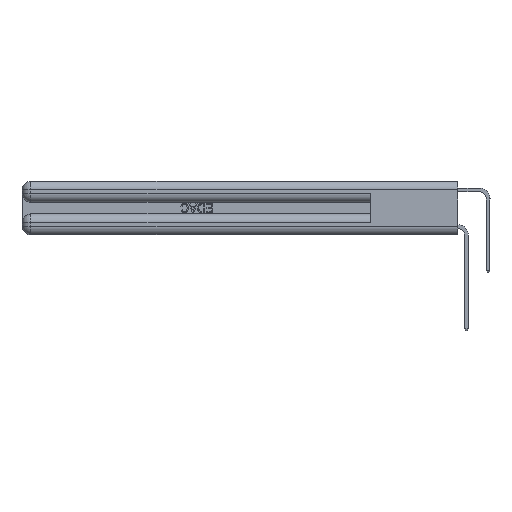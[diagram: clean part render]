
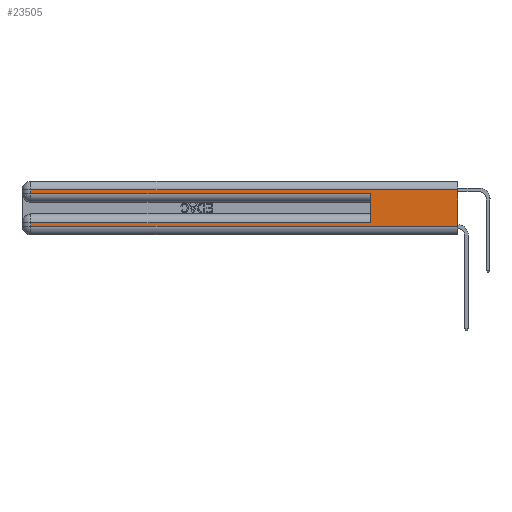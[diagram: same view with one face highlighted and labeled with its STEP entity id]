
A CAD part, left-side view. The second image highlights one B-rep face of the part: STEP entity #23505.
In plain terms, the highlighted planar face has unit normal (-1, 0, 0).
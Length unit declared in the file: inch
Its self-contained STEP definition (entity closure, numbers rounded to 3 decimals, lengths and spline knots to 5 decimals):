
#149 = EDGE_CURVE ( 'NONE', #17727, #10473, #27655, .T. ) ;
#1039 = VERTEX_POINT ( 'NONE', #12734 ) ;
#1341 = DIRECTION ( 'NONE',  ( 0., 0., 1. ) ) ;
#1734 = EDGE_CURVE ( 'NONE', #2657, #15952, #3067, .T. ) ;
#2657 = VERTEX_POINT ( 'NONE', #11048 ) ;
#2810 = LINE ( 'NONE', #22873, #22213 ) ;
#3067 = LINE ( 'NONE', #11424, #16205 ) ;
#3085 = ORIENTED_EDGE ( 'NONE', *, *, #10022, .T. ) ;
#3217 = ORIENTED_EDGE ( 'NONE', *, *, #21176, .T. ) ;
#3412 = ORIENTED_EDGE ( 'NONE', *, *, #6904, .T. ) ;
#5323 = CARTESIAN_POINT ( 'NONE',  ( 0., 0., 0.37 ) ) ;
#5918 = EDGE_CURVE ( 'NONE', #29968, #7331, #22609, .T. ) ;
#6904 = EDGE_CURVE ( 'NONE', #29411, #17727, #2810, .T. ) ;
#6966 = CARTESIAN_POINT ( 'NONE',  ( 0., 2.94, 0.06 ) ) ;
#7202 = CARTESIAN_POINT ( 'NONE',  ( 0., 2.94, 0.37 ) ) ;
#7331 = VERTEX_POINT ( 'NONE', #10230 ) ;
#7752 = VECTOR ( 'NONE', #16326, 39.37008 ) ;
#8032 = DIRECTION ( 'NONE',  ( 0., 1., 0. ) ) ;
#8262 = DIRECTION ( 'NONE',  ( 0., 1., 0. ) ) ;
#9708 = ORIENTED_EDGE ( 'NONE', *, *, #1734, .T. ) ;
#9719 = CARTESIAN_POINT ( 'NONE',  ( 0., 2.94, 0.285 ) ) ;
#10022 = EDGE_CURVE ( 'NONE', #15952, #1039, #27186, .T. ) ;
#10230 = CARTESIAN_POINT ( 'NONE',  ( 0., 0.6, 0.285 ) ) ;
#10473 = VERTEX_POINT ( 'NONE', #9719 ) ;
#10635 = CARTESIAN_POINT ( 'NONE',  ( 0., 0.6, 0.145 ) ) ;
#10859 = VECTOR ( 'NONE', #1341, 39.37008 ) ;
#11048 = CARTESIAN_POINT ( 'NONE',  ( 0., 2.94, 0.085 ) ) ;
#11076 = CARTESIAN_POINT ( 'NONE',  ( 0., 0., 0.06 ) ) ;
#11424 = CARTESIAN_POINT ( 'NONE',  ( 0., 2.94, 0.37 ) ) ;
#12734 = CARTESIAN_POINT ( 'NONE',  ( 0., 0., 0.06 ) ) ;
#14505 = PLANE ( 'NONE',  #25979 ) ;
#14578 = EDGE_LOOP ( 'NONE', ( #15600, #3412, #15776, #3217, #28847, #24813, #9708, #3085 ) ) ;
#14711 = DIRECTION ( 'NONE',  ( 1., 0., 0. ) ) ;
#14730 = CARTESIAN_POINT ( 'NONE',  ( 0., 0., 0.37 ) ) ;
#15600 = ORIENTED_EDGE ( 'NONE', *, *, #21823, .F. ) ;
#15776 = ORIENTED_EDGE ( 'NONE', *, *, #149, .T. ) ;
#15952 = VERTEX_POINT ( 'NONE', #6966 ) ;
#16045 = CARTESIAN_POINT ( 'NONE',  ( 0., 0., 0.31 ) ) ;
#16152 = LINE ( 'NONE', #29130, #29657 ) ;
#16205 = VECTOR ( 'NONE', #23136, 39.37008 ) ;
#16326 = DIRECTION ( 'NONE',  ( 0., -1., 0. ) ) ;
#17583 = VECTOR ( 'NONE', #26133, 39.37008 ) ;
#17727 = VERTEX_POINT ( 'NONE', #28388 ) ;
#17925 = LINE ( 'NONE', #14730, #27841 ) ;
#19330 = DIRECTION ( 'NONE',  ( 0., 0., -1. ) ) ;
#20706 = EDGE_CURVE ( 'NONE', #29968, #2657, #16152, .T. ) ;
#21133 = CARTESIAN_POINT ( 'NONE',  ( 0., 0.6, 0.085 ) ) ;
#21176 = EDGE_CURVE ( 'NONE', #10473, #7331, #26008, .T. ) ;
#21823 = EDGE_CURVE ( 'NONE', #29411, #1039, #17925, .T. ) ;
#22213 = VECTOR ( 'NONE', #8032, 39.37008 ) ;
#22609 = LINE ( 'NONE', #10635, #10859 ) ;
#22873 = CARTESIAN_POINT ( 'NONE',  ( 0., 0., 0.31 ) ) ;
#23136 = DIRECTION ( 'NONE',  ( 0., 0., -1. ) ) ;
#23505 = ADVANCED_FACE ( 'NONE', ( #23758 ), #14505, .F. ) ;
#23659 = VECTOR ( 'NONE', #28151, 39.37008 ) ;
#23758 = FACE_OUTER_BOUND ( 'NONE', #14578, .T. ) ;
#23943 = DIRECTION ( 'NONE',  ( 0., 0., -1. ) ) ;
#24813 = ORIENTED_EDGE ( 'NONE', *, *, #20706, .T. ) ;
#25979 = AXIS2_PLACEMENT_3D ( 'NONE', #5323, #14711, #23943 ) ;
#26008 = LINE ( 'NONE', #28162, #17583 ) ;
#26133 = DIRECTION ( 'NONE',  ( 0., -1., 0. ) ) ;
#27186 = LINE ( 'NONE', #11076, #7752 ) ;
#27655 = LINE ( 'NONE', #7202, #23659 ) ;
#27841 = VECTOR ( 'NONE', #19330, 39.37008 ) ;
#28151 = DIRECTION ( 'NONE',  ( 0., 0., -1. ) ) ;
#28162 = CARTESIAN_POINT ( 'NONE',  ( 0., 0., 0.285 ) ) ;
#28388 = CARTESIAN_POINT ( 'NONE',  ( 0., 2.94, 0.31 ) ) ;
#28847 = ORIENTED_EDGE ( 'NONE', *, *, #5918, .F. ) ;
#29130 = CARTESIAN_POINT ( 'NONE',  ( 0., 0., 0.085 ) ) ;
#29411 = VERTEX_POINT ( 'NONE', #16045 ) ;
#29657 = VECTOR ( 'NONE', #8262, 39.37008 ) ;
#29968 = VERTEX_POINT ( 'NONE', #21133 ) ;
